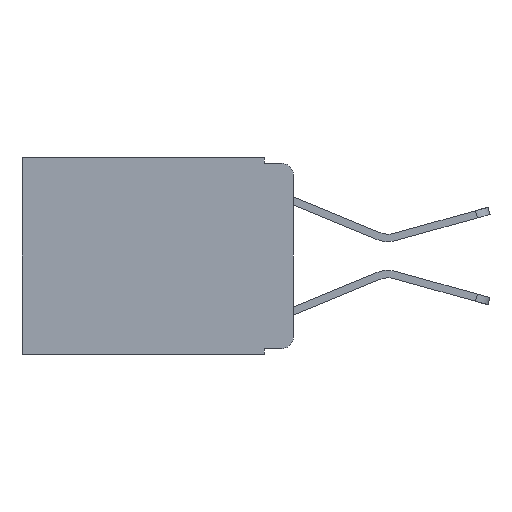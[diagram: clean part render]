
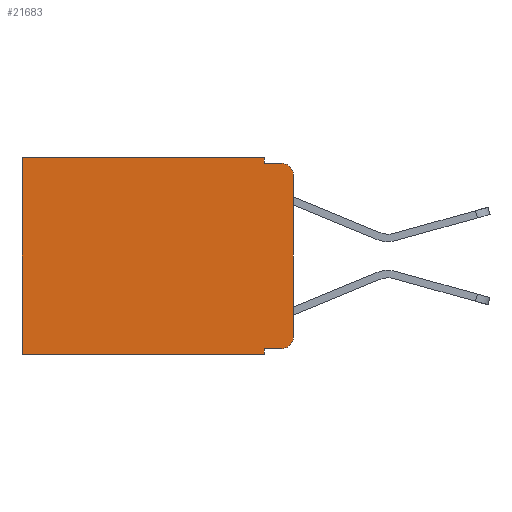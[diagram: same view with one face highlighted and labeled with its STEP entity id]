
A CAD part, left-side view. The second image highlights one B-rep face of the part: STEP entity #21683.
In plain terms, the highlighted planar face has unit normal (-1, 0, 0).
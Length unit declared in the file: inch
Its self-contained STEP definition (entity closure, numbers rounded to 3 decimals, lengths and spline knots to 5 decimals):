
#22 = DIRECTION ( 'NONE',  ( 0., 0., -1. ) ) ;
#94 = CIRCLE ( 'NONE', #7270, 0.02 ) ;
#235 = AXIS2_PLACEMENT_3D ( 'NONE', #20421, #7298, #5783 ) ;
#262 = EDGE_CURVE ( 'NONE', #4335, #19562, #8277, .T. ) ;
#459 = CARTESIAN_POINT ( 'NONE',  ( 0.298, 0.051, 0. ) ) ;
#1073 = LINE ( 'NONE', #23169, #20071 ) ;
#1276 = EDGE_CURVE ( 'NONE', #16021, #12732, #21909, .T. ) ;
#1740 = LINE ( 'NONE', #22124, #20673 ) ;
#1872 = CARTESIAN_POINT ( 'NONE',  ( 0.298, 0., -0.343 ) ) ;
#1982 = ORIENTED_EDGE ( 'NONE', *, *, #16979, .T. ) ;
#3197 = EDGE_CURVE ( 'NONE', #15332, #12732, #10136, .T. ) ;
#3740 = CARTESIAN_POINT ( 'NONE',  ( 0.298, 0.051, 0. ) ) ;
#4008 = EDGE_CURVE ( 'NONE', #11482, #4335, #17963, .T. ) ;
#4335 = VERTEX_POINT ( 'NONE', #12693 ) ;
#4563 = CARTESIAN_POINT ( 'NONE',  ( 0.298, 0.051, -0.01 ) ) ;
#4637 = CARTESIAN_POINT ( 'NONE',  ( 0.298, 0.473, -0.343 ) ) ;
#4757 = CARTESIAN_POINT ( 'NONE',  ( 0.298, 0.02, -0.333 ) ) ;
#5148 = LINE ( 'NONE', #6801, #10117 ) ;
#5164 = VECTOR ( 'NONE', #14122, 39.37008 ) ;
#5242 = DIRECTION ( 'NONE',  ( 0., 1., 0. ) ) ;
#5783 = DIRECTION ( 'NONE',  ( 0., 0., -1. ) ) ;
#6298 = EDGE_CURVE ( 'NONE', #19531, #15150, #18969, .T. ) ;
#6644 = CARTESIAN_POINT ( 'NONE',  ( 0.298, 0., -0.03 ) ) ;
#6801 = CARTESIAN_POINT ( 'NONE',  ( 0.298, 0.051, -0.333 ) ) ;
#6913 = CARTESIAN_POINT ( 'NONE',  ( 0.298, 0., 0. ) ) ;
#7131 = ORIENTED_EDGE ( 'NONE', *, *, #4008, .F. ) ;
#7270 = AXIS2_PLACEMENT_3D ( 'NONE', #22034, #11420, #22 ) ;
#7298 = DIRECTION ( 'NONE',  ( -1., 0., 0. ) ) ;
#7375 = CARTESIAN_POINT ( 'NONE',  ( 0.298, 0.051, -0.01 ) ) ;
#7703 = VECTOR ( 'NONE', #23349, 39.37008 ) ;
#7872 = CARTESIAN_POINT ( 'NONE',  ( 0.298, 0.02, -0.01 ) ) ;
#8277 = LINE ( 'NONE', #1872, #7703 ) ;
#8802 = VERTEX_POINT ( 'NONE', #3740 ) ;
#9230 = DIRECTION ( 'NONE',  ( 0., -1., 0. ) ) ;
#9362 = CARTESIAN_POINT ( 'NONE',  ( 0.298, 0., -0.313 ) ) ;
#9696 = DIRECTION ( 'NONE',  ( 0., 0., -1. ) ) ;
#9971 = CARTESIAN_POINT ( 'NONE',  ( 0.298, 0.473, 0. ) ) ;
#10117 = VECTOR ( 'NONE', #17605, 39.37008 ) ;
#10136 = LINE ( 'NONE', #6913, #5164 ) ;
#10863 = FACE_OUTER_BOUND ( 'NONE', #22128, .T. ) ;
#11367 = EDGE_CURVE ( 'NONE', #15332, #15150, #94, .T. ) ;
#11420 = DIRECTION ( 'NONE',  ( -1., 0., 0. ) ) ;
#11482 = VERTEX_POINT ( 'NONE', #17055 ) ;
#12143 = DIRECTION ( 'NONE',  ( 0., 0., -1. ) ) ;
#12693 = CARTESIAN_POINT ( 'NONE',  ( 0.298, 0.051, -0.343 ) ) ;
#12732 = VERTEX_POINT ( 'NONE', #9362 ) ;
#13517 = ORIENTED_EDGE ( 'NONE', *, *, #3197, .F. ) ;
#14122 = DIRECTION ( 'NONE',  ( 0., 0., -1. ) ) ;
#14220 = VECTOR ( 'NONE', #9230, 39.37008 ) ;
#14295 = EDGE_CURVE ( 'NONE', #11482, #16021, #5148, .T. ) ;
#15150 = VERTEX_POINT ( 'NONE', #7872 ) ;
#15332 = VERTEX_POINT ( 'NONE', #6644 ) ;
#15609 = ORIENTED_EDGE ( 'NONE', *, *, #6298, .F. ) ;
#15643 = CARTESIAN_POINT ( 'NONE',  ( 0.298, 0., 0. ) ) ;
#15759 = EDGE_CURVE ( 'NONE', #8802, #19531, #1740, .T. ) ;
#16021 = VERTEX_POINT ( 'NONE', #4757 ) ;
#16238 = ORIENTED_EDGE ( 'NONE', *, *, #11367, .T. ) ;
#16646 = EDGE_CURVE ( 'NONE', #8802, #19221, #1073, .T. ) ;
#16979 = EDGE_CURVE ( 'NONE', #19221, #19562, #22776, .T. ) ;
#17055 = CARTESIAN_POINT ( 'NONE',  ( 0.298, 0.051, -0.333 ) ) ;
#17304 = ORIENTED_EDGE ( 'NONE', *, *, #1276, .T. ) ;
#17356 = ORIENTED_EDGE ( 'NONE', *, *, #16646, .T. ) ;
#17403 = VECTOR ( 'NONE', #22234, 39.37008 ) ;
#17550 = VECTOR ( 'NONE', #20645, 39.37008 ) ;
#17605 = DIRECTION ( 'NONE',  ( 0., -1., 0. ) ) ;
#17963 = LINE ( 'NONE', #459, #17403 ) ;
#18471 = ORIENTED_EDGE ( 'NONE', *, *, #262, .F. ) ;
#18969 = LINE ( 'NONE', #7375, #14220 ) ;
#19032 = ORIENTED_EDGE ( 'NONE', *, *, #14295, .T. ) ;
#19221 = VERTEX_POINT ( 'NONE', #21793 ) ;
#19531 = VERTEX_POINT ( 'NONE', #4563 ) ;
#19562 = VERTEX_POINT ( 'NONE', #4637 ) ;
#19629 = AXIS2_PLACEMENT_3D ( 'NONE', #15643, #22730, #12143 ) ;
#20071 = VECTOR ( 'NONE', #5242, 39.37008 ) ;
#20421 = CARTESIAN_POINT ( 'NONE',  ( 0.298, 0.02, -0.313 ) ) ;
#20645 = DIRECTION ( 'NONE',  ( 0., 0., -1. ) ) ;
#20673 = VECTOR ( 'NONE', #9696, 39.37008 ) ;
#20936 = ORIENTED_EDGE ( 'NONE', *, *, #15759, .F. ) ;
#20987 = PLANE ( 'NONE',  #19629 ) ;
#21683 = ADVANCED_FACE ( 'NONE', ( #10863 ), #20987, .F. ) ;
#21793 = CARTESIAN_POINT ( 'NONE',  ( 0.298, 0.473, 0. ) ) ;
#21909 = CIRCLE ( 'NONE', #235, 0.02 ) ;
#22034 = CARTESIAN_POINT ( 'NONE',  ( 0.298, 0.02, -0.03 ) ) ;
#22124 = CARTESIAN_POINT ( 'NONE',  ( 0.298, 0.051, 0. ) ) ;
#22128 = EDGE_LOOP ( 'NONE', ( #13517, #16238, #15609, #20936, #17356, #1982, #18471, #7131, #19032, #17304 ) ) ;
#22234 = DIRECTION ( 'NONE',  ( 0., 0., -1. ) ) ;
#22730 = DIRECTION ( 'NONE',  ( 1., 0., 0. ) ) ;
#22776 = LINE ( 'NONE', #9971, #17550 ) ;
#23169 = CARTESIAN_POINT ( 'NONE',  ( 0.298, 0., 0. ) ) ;
#23349 = DIRECTION ( 'NONE',  ( 0., 1., 0. ) ) ;
